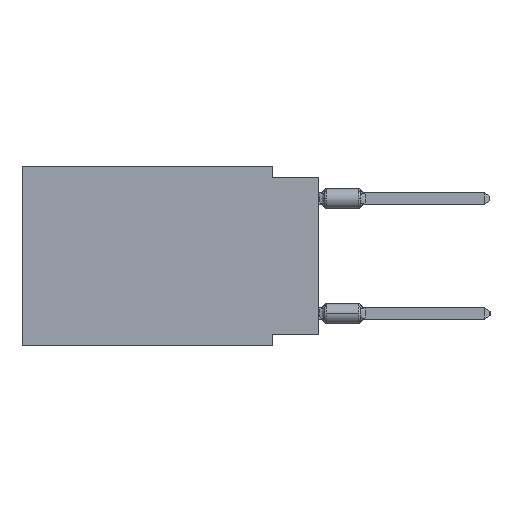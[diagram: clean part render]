
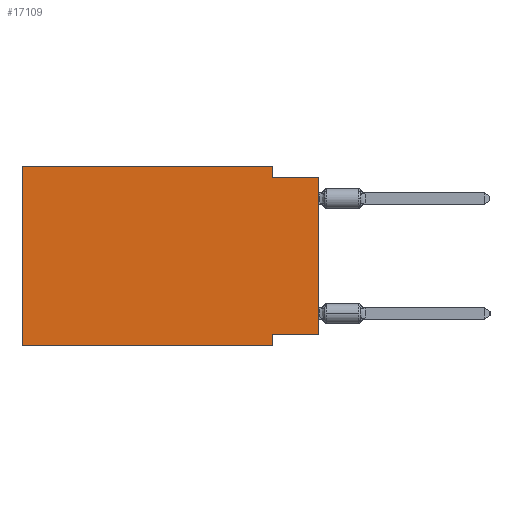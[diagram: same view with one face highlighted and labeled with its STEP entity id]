
A CAD part, left-side view. The second image highlights one B-rep face of the part: STEP entity #17109.
In plain terms, the highlighted planar face has unit normal (-1, 0, 0).
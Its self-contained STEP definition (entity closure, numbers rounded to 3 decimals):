
#9 = CARTESIAN_POINT ( 'NONE',  ( 0., 0., -9.271 ) ) ;
#359 = VERTEX_POINT ( 'NONE', #33339 ) ;
#768 = EDGE_CURVE ( 'NONE', #7506, #11272, #1189, .T. ) ;
#1189 = LINE ( 'NONE', #9158, #4875 ) ;
#2938 = VERTEX_POINT ( 'NONE', #9 ) ;
#4168 = ORIENTED_EDGE ( 'NONE', *, *, #22950, .F. ) ;
#4875 = VECTOR ( 'NONE', #29628, 1000. ) ;
#5215 = CARTESIAN_POINT ( 'NONE',  ( 0., 16.383, 0. ) ) ;
#5382 = LINE ( 'NONE', #20052, #24962 ) ;
#6269 = EDGE_CURVE ( 'NONE', #359, #34462, #12528, .T. ) ;
#6515 = VECTOR ( 'NONE', #23722, 1000. ) ;
#7506 = VERTEX_POINT ( 'NONE', #30438 ) ;
#8448 = CARTESIAN_POINT ( 'NONE',  ( 0., 16.383, -9.906 ) ) ;
#9158 = CARTESIAN_POINT ( 'NONE',  ( 0., 2.54, -9.906 ) ) ;
#9159 = ORIENTED_EDGE ( 'NONE', *, *, #6269, .F. ) ;
#9529 = ORIENTED_EDGE ( 'NONE', *, *, #36215, .F. ) ;
#11187 = DIRECTION ( 'NONE',  ( 1., 0., 0. ) ) ;
#11189 = LINE ( 'NONE', #34755, #35986 ) ;
#11272 = VERTEX_POINT ( 'NONE', #17595 ) ;
#11340 = LINE ( 'NONE', #8448, #26516 ) ;
#11368 = CARTESIAN_POINT ( 'NONE',  ( 0., 16.383, -9.906 ) ) ;
#12528 = LINE ( 'NONE', #36302, #21089 ) ;
#12925 = VERTEX_POINT ( 'NONE', #11368 ) ;
#13129 = VECTOR ( 'NONE', #22298, 1000. ) ;
#14058 = EDGE_CURVE ( 'NONE', #2938, #34462, #32811, .T. ) ;
#14465 = PLANE ( 'NONE',  #20808 ) ;
#14579 = CARTESIAN_POINT ( 'NONE',  ( 0., 2.54, 0. ) ) ;
#16321 = LINE ( 'NONE', #25202, #13129 ) ;
#16779 = LINE ( 'NONE', #25852, #31441 ) ;
#17109 = ADVANCED_FACE ( 'NONE', ( #29145 ), #14465, .F. ) ;
#17341 = DIRECTION ( 'NONE',  ( 0., 1., 0. ) ) ;
#17595 = CARTESIAN_POINT ( 'NONE',  ( 0., 2.54, -9.906 ) ) ;
#19052 = EDGE_CURVE ( 'NONE', #26415, #359, #11189, .T. ) ;
#19845 = DIRECTION ( 'NONE',  ( 0., -1., 0. ) ) ;
#20052 = CARTESIAN_POINT ( 'NONE',  ( 0., 0., -9.271 ) ) ;
#20267 = DIRECTION ( 'NONE',  ( 0., 0., -1. ) ) ;
#20278 = CARTESIAN_POINT ( 'NONE',  ( 0., 16.383, 0. ) ) ;
#20808 = AXIS2_PLACEMENT_3D ( 'NONE', #5215, #11187, #28782 ) ;
#21089 = VECTOR ( 'NONE', #30496, 1000. ) ;
#22298 = DIRECTION ( 'NONE',  ( 0., -1., 0. ) ) ;
#22343 = ORIENTED_EDGE ( 'NONE', *, *, #19052, .F. ) ;
#22763 = DIRECTION ( 'NONE',  ( 0., 0., 1. ) ) ;
#22950 = EDGE_CURVE ( 'NONE', #2938, #7506, #5382, .T. ) ;
#23722 = DIRECTION ( 'NONE',  ( 0., 0., 1. ) ) ;
#24962 = VECTOR ( 'NONE', #17341, 1000. ) ;
#25202 = CARTESIAN_POINT ( 'NONE',  ( 0., 16.383, 0. ) ) ;
#25852 = CARTESIAN_POINT ( 'NONE',  ( 0., 16.383, 0. ) ) ;
#26415 = VERTEX_POINT ( 'NONE', #14579 ) ;
#26516 = VECTOR ( 'NONE', #19845, 1000. ) ;
#26873 = ORIENTED_EDGE ( 'NONE', *, *, #27558, .F. ) ;
#27343 = EDGE_LOOP ( 'NONE', ( #36463, #9159, #22343, #26873, #9529, #36055, #37980, #4168 ) ) ;
#27558 = EDGE_CURVE ( 'NONE', #30177, #26415, #16321, .T. ) ;
#28782 = DIRECTION ( 'NONE',  ( 0., 0., -1. ) ) ;
#29145 = FACE_OUTER_BOUND ( 'NONE', #27343, .T. ) ;
#29628 = DIRECTION ( 'NONE',  ( 0., 0., -1. ) ) ;
#30177 = VERTEX_POINT ( 'NONE', #20278 ) ;
#30438 = CARTESIAN_POINT ( 'NONE',  ( 0., 2.54, -9.271 ) ) ;
#30496 = DIRECTION ( 'NONE',  ( 0., -1., 0. ) ) ;
#31441 = VECTOR ( 'NONE', #22763, 1000. ) ;
#32419 = CARTESIAN_POINT ( 'NONE',  ( 0., 0., 0. ) ) ;
#32811 = LINE ( 'NONE', #32419, #6515 ) ;
#33339 = CARTESIAN_POINT ( 'NONE',  ( 0., 2.54, -0.635 ) ) ;
#33386 = EDGE_CURVE ( 'NONE', #12925, #11272, #11340, .T. ) ;
#34462 = VERTEX_POINT ( 'NONE', #34968 ) ;
#34755 = CARTESIAN_POINT ( 'NONE',  ( 0., 2.54, 0. ) ) ;
#34968 = CARTESIAN_POINT ( 'NONE',  ( 0., 0., -0.635 ) ) ;
#35986 = VECTOR ( 'NONE', #20267, 1000. ) ;
#36055 = ORIENTED_EDGE ( 'NONE', *, *, #33386, .T. ) ;
#36215 = EDGE_CURVE ( 'NONE', #12925, #30177, #16779, .T. ) ;
#36302 = CARTESIAN_POINT ( 'NONE',  ( 0., 0., -0.635 ) ) ;
#36463 = ORIENTED_EDGE ( 'NONE', *, *, #14058, .T. ) ;
#37980 = ORIENTED_EDGE ( 'NONE', *, *, #768, .F. ) ;
